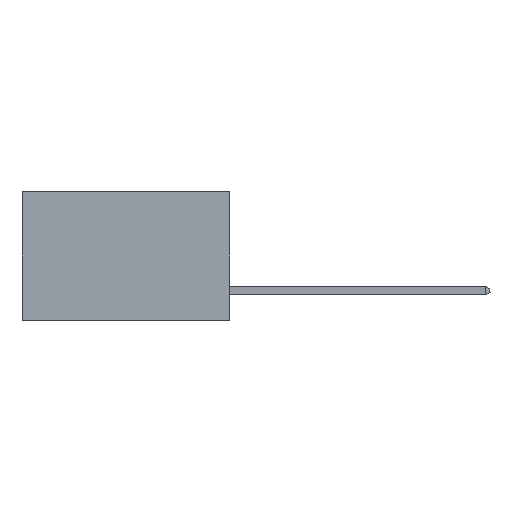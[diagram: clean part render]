
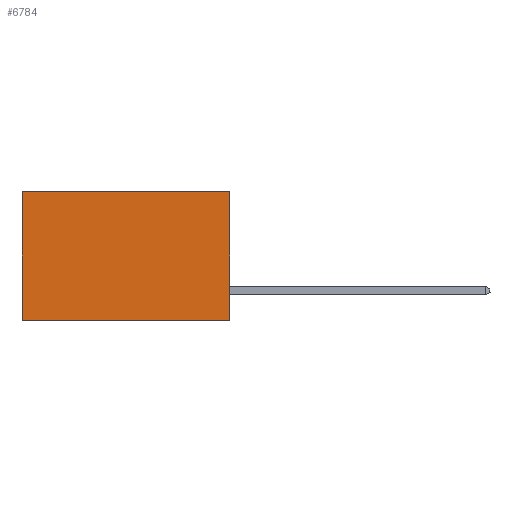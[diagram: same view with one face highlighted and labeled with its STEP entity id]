
A CAD part, left-side view. The second image highlights one B-rep face of the part: STEP entity #6784.
In plain terms, the highlighted planar face has unit normal (-1, 0, 0).
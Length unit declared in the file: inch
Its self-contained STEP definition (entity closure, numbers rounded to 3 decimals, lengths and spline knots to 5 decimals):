
#146 = CARTESIAN_POINT ( 'NONE',  ( 0.298, 0., 0. ) ) ;
#219 = VERTEX_POINT ( 'NONE', #9175 ) ;
#2588 = AXIS2_PLACEMENT_3D ( 'NONE', #17257, #8203, #10424 ) ;
#5291 = EDGE_CURVE ( 'NONE', #17145, #219, #26466, .T. ) ;
#5724 = EDGE_CURVE ( 'NONE', #219, #23297, #11329, .T. ) ;
#5984 = PLANE ( 'NONE',  #2588 ) ;
#6438 = FACE_OUTER_BOUND ( 'NONE', #6512, .T. ) ;
#6512 = EDGE_LOOP ( 'NONE', ( #23029, #24086, #18313, #14415 ) ) ;
#6521 = DIRECTION ( 'NONE',  ( 0., 1., 0. ) ) ;
#6784 = ADVANCED_FACE ( 'NONE', ( #6438 ), #5984, .F. ) ;
#7693 = CARTESIAN_POINT ( 'NONE',  ( 0.298, 0.6, 0. ) ) ;
#8203 = DIRECTION ( 'NONE',  ( 1., 0., 0. ) ) ;
#8489 = CARTESIAN_POINT ( 'NONE',  ( 0.298, 0.6, 0. ) ) ;
#9175 = CARTESIAN_POINT ( 'NONE',  ( 0.298, 0., -0.37 ) ) ;
#10424 = DIRECTION ( 'NONE',  ( 0., 0., -1. ) ) ;
#11329 = LINE ( 'NONE', #23254, #14775 ) ;
#12468 = VECTOR ( 'NONE', #6521, 39.37008 ) ;
#12882 = EDGE_CURVE ( 'NONE', #17145, #27938, #15559, .T. ) ;
#13197 = DIRECTION ( 'NONE',  ( 0., 0., -1. ) ) ;
#14415 = ORIENTED_EDGE ( 'NONE', *, *, #12882, .T. ) ;
#14775 = VECTOR ( 'NONE', #20792, 39.37008 ) ;
#15014 = CARTESIAN_POINT ( 'NONE',  ( 0.298, 0., 0. ) ) ;
#15559 = LINE ( 'NONE', #27995, #12468 ) ;
#17145 = VERTEX_POINT ( 'NONE', #146 ) ;
#17257 = CARTESIAN_POINT ( 'NONE',  ( 0.298, 0., 0. ) ) ;
#17400 = VECTOR ( 'NONE', #23812, 39.37008 ) ;
#17559 = VECTOR ( 'NONE', #13197, 39.37008 ) ;
#17690 = CARTESIAN_POINT ( 'NONE',  ( 0.298, 0.6, -0.37 ) ) ;
#18233 = EDGE_CURVE ( 'NONE', #27938, #23297, #18395, .T. ) ;
#18313 = ORIENTED_EDGE ( 'NONE', *, *, #5291, .F. ) ;
#18395 = LINE ( 'NONE', #8489, #17400 ) ;
#20792 = DIRECTION ( 'NONE',  ( 0., 1., 0. ) ) ;
#23029 = ORIENTED_EDGE ( 'NONE', *, *, #18233, .T. ) ;
#23254 = CARTESIAN_POINT ( 'NONE',  ( 0.298, 0., -0.37 ) ) ;
#23297 = VERTEX_POINT ( 'NONE', #17690 ) ;
#23812 = DIRECTION ( 'NONE',  ( 0., 0., -1. ) ) ;
#24086 = ORIENTED_EDGE ( 'NONE', *, *, #5724, .F. ) ;
#26466 = LINE ( 'NONE', #15014, #17559 ) ;
#27938 = VERTEX_POINT ( 'NONE', #7693 ) ;
#27995 = CARTESIAN_POINT ( 'NONE',  ( 0.298, 0., 0. ) ) ;
